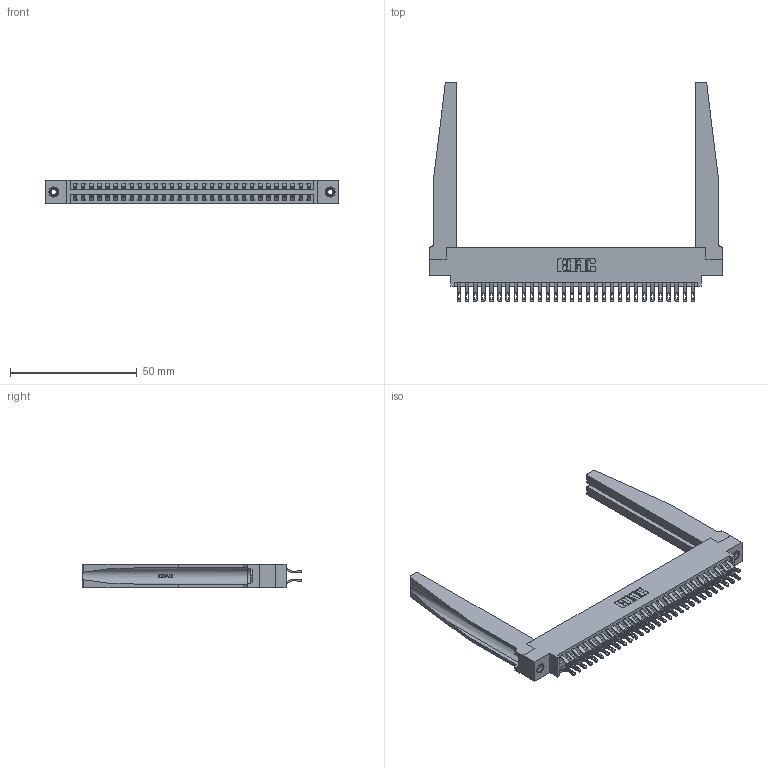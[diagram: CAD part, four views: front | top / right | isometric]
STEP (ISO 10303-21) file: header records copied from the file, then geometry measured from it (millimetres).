
FILE_DESCRIPTION (( 'STEP AP203' ), '1' );
FILE_NAME ('346-060-555-878.STEP', '2022-05-21T11:58:08', ( '' ), ( '' ), 'SwSTEP 2.0', 'SolidWorks 2020', '' );
FILE_SCHEMA (( 'CONFIG_CONTROL_DESIGN' ));
Length unit declared in the file: inch
Products named in the file (5): 346-220-078_345-220-078; 346-060-555-878; 345-250-001_345-250-001-102; 346 Part_0.170 Offset - 0.156 Dia-TH; 345-292-001_555 Tail
Assembly tree (65 placements, depth 2):
  346-060-555-878
    346 Part_0.170 Offset - 0.156 Dia-TH
    345-292-001_555 Tail  x60
    346-220-078_345-220-078  x2
    345-250-001_345-250-001-102  x2
Bounding box: 115.82 x 86.74 x 9.4 mm (x, y, z)
Volume: 18111.3 mm3; surface area: 22581.9 mm2
Topology: 65 solids, 65 shells, 3854 faces, 11965 edges, 7966 vertices
Faces by surface type: plane 2216, cylinder 1586, bspline 36, cone 12, torus 4
Entity records: 26816 total; most frequent: CARTESIAN_POINT 5415, ORIENTED_EDGE 4206, DIRECTION 3777, EDGE_CURVE 2103, VECTOR 1737, LINE 1737, VERTEX_POINT 1396, AXIS2_PLACEMENT_3D 1020
